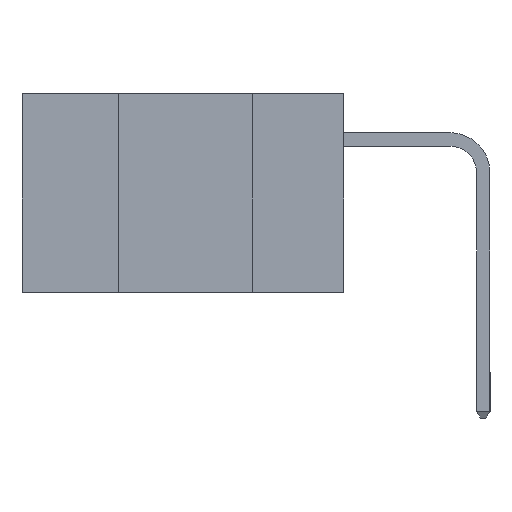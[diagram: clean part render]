
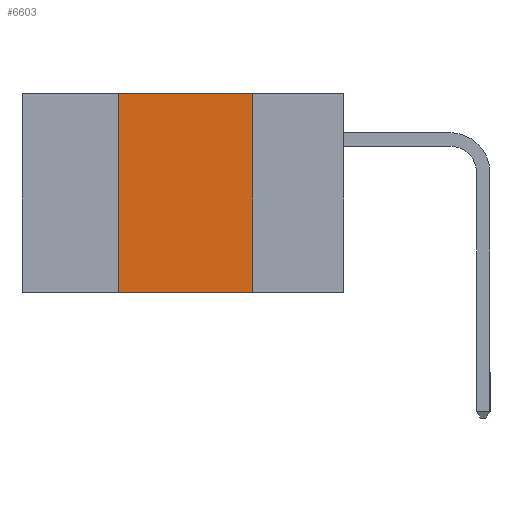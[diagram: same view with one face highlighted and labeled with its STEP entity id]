
A CAD part, left-side view. The second image highlights one B-rep face of the part: STEP entity #6603.
In plain terms, the highlighted planar face has unit normal (-1, 0, 0).
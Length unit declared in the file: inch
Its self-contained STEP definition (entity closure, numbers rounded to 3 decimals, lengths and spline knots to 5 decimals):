
#471 = CARTESIAN_POINT ( 'NONE',  ( 0., 0.42, 0. ) ) ;
#590 = EDGE_CURVE ( 'NONE', #4662, #7006, #8142, .T. ) ;
#660 = DIRECTION ( 'NONE',  ( 0., -1., 0. ) ) ;
#770 = CARTESIAN_POINT ( 'NONE',  ( 0., 0.17, 0. ) ) ;
#890 = LINE ( 'NONE', #7835, #6051 ) ;
#897 = CARTESIAN_POINT ( 'NONE',  ( 0., 0.6, -0.37 ) ) ;
#1732 = VECTOR ( 'NONE', #5816, 39.37008 ) ;
#1794 = ORIENTED_EDGE ( 'NONE', *, *, #3653, .F. ) ;
#2007 = DIRECTION ( 'NONE',  ( 0., 0., -1. ) ) ;
#2402 = VECTOR ( 'NONE', #660, 39.37008 ) ;
#2437 = DIRECTION ( 'NONE',  ( 0., 0., -1. ) ) ;
#2597 = LINE ( 'NONE', #7379, #4824 ) ;
#2701 = ORIENTED_EDGE ( 'NONE', *, *, #590, .F. ) ;
#3422 = DIRECTION ( 'NONE',  ( 1., 0., 0. ) ) ;
#3653 = EDGE_CURVE ( 'NONE', #7006, #8374, #2597, .T. ) ;
#3723 = AXIS2_PLACEMENT_3D ( 'NONE', #7667, #3422, #2007 ) ;
#4033 = VERTEX_POINT ( 'NONE', #6959 ) ;
#4048 = CARTESIAN_POINT ( 'NONE',  ( 0., 0.6, 0. ) ) ;
#4496 = ORIENTED_EDGE ( 'NONE', *, *, #5329, .T. ) ;
#4655 = LINE ( 'NONE', #897, #1732 ) ;
#4662 = VERTEX_POINT ( 'NONE', #471 ) ;
#4824 = VECTOR ( 'NONE', #2437, 39.37008 ) ;
#5329 = EDGE_CURVE ( 'NONE', #4033, #8374, #4655, .T. ) ;
#5816 = DIRECTION ( 'NONE',  ( 0., -1., 0. ) ) ;
#5829 = ORIENTED_EDGE ( 'NONE', *, *, #8141, .F. ) ;
#6051 = VECTOR ( 'NONE', #7806, 39.37008 ) ;
#6423 = FACE_OUTER_BOUND ( 'NONE', #7030, .T. ) ;
#6603 = ADVANCED_FACE ( 'NONE', ( #6423 ), #7033, .F. ) ;
#6719 = CARTESIAN_POINT ( 'NONE',  ( 0., 0.17, -0.37 ) ) ;
#6959 = CARTESIAN_POINT ( 'NONE',  ( 0., 0.42, -0.37 ) ) ;
#7006 = VERTEX_POINT ( 'NONE', #770 ) ;
#7030 = EDGE_LOOP ( 'NONE', ( #1794, #2701, #5829, #4496 ) ) ;
#7033 = PLANE ( 'NONE',  #3723 ) ;
#7379 = CARTESIAN_POINT ( 'NONE',  ( 0., 0.17, 0. ) ) ;
#7667 = CARTESIAN_POINT ( 'NONE',  ( 0., 0.6, 0. ) ) ;
#7806 = DIRECTION ( 'NONE',  ( 0., 0., 1. ) ) ;
#7835 = CARTESIAN_POINT ( 'NONE',  ( 0., 0.42, 0. ) ) ;
#8141 = EDGE_CURVE ( 'NONE', #4033, #4662, #890, .T. ) ;
#8142 = LINE ( 'NONE', #4048, #2402 ) ;
#8374 = VERTEX_POINT ( 'NONE', #6719 ) ;
